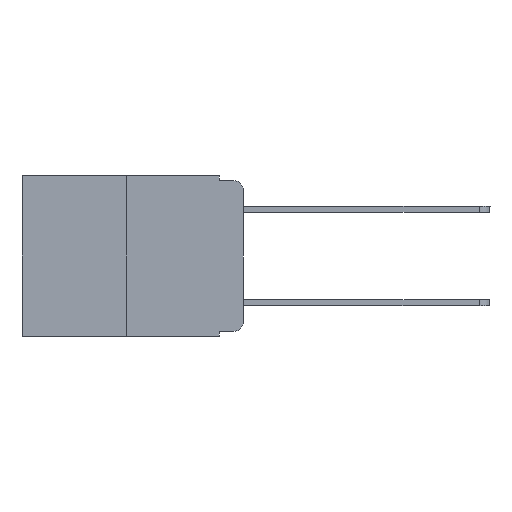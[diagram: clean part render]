
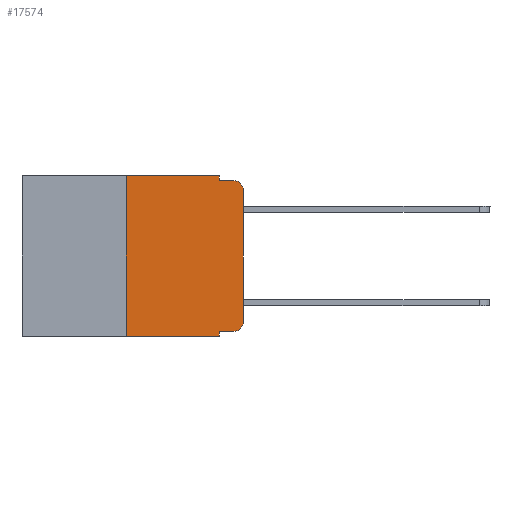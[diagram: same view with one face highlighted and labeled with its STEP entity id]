
A CAD part, left-side view. The second image highlights one B-rep face of the part: STEP entity #17574.
In plain terms, the highlighted planar face has unit normal (-1, 0, 0).
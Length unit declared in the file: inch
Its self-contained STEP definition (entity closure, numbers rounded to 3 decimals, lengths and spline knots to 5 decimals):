
#331 = EDGE_CURVE ( 'NONE', #4252, #5322, #2284, .T. ) ;
#807 = CARTESIAN_POINT ( 'NONE',  ( 0., 0.25, 0. ) ) ;
#851 = EDGE_CURVE ( 'NONE', #12747, #7354, #23218, .T. ) ;
#2124 = VERTEX_POINT ( 'NONE', #18488 ) ;
#2284 = LINE ( 'NONE', #20363, #13261 ) ;
#2447 = DIRECTION ( 'NONE',  ( 1., 0., 0. ) ) ;
#3952 = CARTESIAN_POINT ( 'NONE',  ( 0., 0.473, 0. ) ) ;
#4152 = EDGE_CURVE ( 'NONE', #25051, #7354, #22357, .T. ) ;
#4252 = VERTEX_POINT ( 'NONE', #8072 ) ;
#4361 = ORIENTED_EDGE ( 'NONE', *, *, #22997, .T. ) ;
#4567 = CIRCLE ( 'NONE', #19633, 0.02 ) ;
#4842 = ORIENTED_EDGE ( 'NONE', *, *, #851, .F. ) ;
#4973 = LINE ( 'NONE', #807, #24078 ) ;
#5035 = EDGE_CURVE ( 'NONE', #2124, #22050, #17595, .T. ) ;
#5322 = VERTEX_POINT ( 'NONE', #6813 ) ;
#5369 = DIRECTION ( 'NONE',  ( 0., -1., 0. ) ) ;
#6044 = CARTESIAN_POINT ( 'NONE',  ( 0., 0.051, -0.333 ) ) ;
#6506 = VERTEX_POINT ( 'NONE', #17336 ) ;
#6664 = VERTEX_POINT ( 'NONE', #6044 ) ;
#6665 = DIRECTION ( 'NONE',  ( 0., 0., 1. ) ) ;
#6740 = FACE_OUTER_BOUND ( 'NONE', #7889, .T. ) ;
#6813 = CARTESIAN_POINT ( 'NONE',  ( 0., 0.051, -0.343 ) ) ;
#6892 = ORIENTED_EDGE ( 'NONE', *, *, #12674, .F. ) ;
#7354 = VERTEX_POINT ( 'NONE', #19375 ) ;
#7362 = CARTESIAN_POINT ( 'NONE',  ( 0., 0.02, -0.333 ) ) ;
#7423 = DIRECTION ( 'NONE',  ( 0., 0., 1. ) ) ;
#7484 = ORIENTED_EDGE ( 'NONE', *, *, #12134, .F. ) ;
#7503 = VECTOR ( 'NONE', #5369, 39.37008 ) ;
#7889 = EDGE_LOOP ( 'NONE', ( #4361, #16773, #4842, #18980, #21516, #7484, #25048, #6892, #12847, #23120 ) ) ;
#8072 = CARTESIAN_POINT ( 'NONE',  ( 0., 0.25, -0.343 ) ) ;
#8151 = VECTOR ( 'NONE', #14756, 39.37008 ) ;
#8222 = LINE ( 'NONE', #10553, #11292 ) ;
#8453 = EDGE_CURVE ( 'NONE', #6664, #16986, #21256, .T. ) ;
#8575 = CARTESIAN_POINT ( 'NONE',  ( 0., 0.473, 0. ) ) ;
#8596 = CARTESIAN_POINT ( 'NONE',  ( 0., 0.051, 0. ) ) ;
#9507 = VECTOR ( 'NONE', #17309, 39.37008 ) ;
#10553 = CARTESIAN_POINT ( 'NONE',  ( 0., 0.051, 0. ) ) ;
#10653 = DIRECTION ( 'NONE',  ( -1., 0., 0. ) ) ;
#11100 = AXIS2_PLACEMENT_3D ( 'NONE', #8575, #2447, #12362 ) ;
#11216 = EDGE_CURVE ( 'NONE', #22050, #12747, #8222, .T. ) ;
#11217 = DIRECTION ( 'NONE',  ( -1., 0., 0. ) ) ;
#11292 = VECTOR ( 'NONE', #18573, 39.37008 ) ;
#12134 = EDGE_CURVE ( 'NONE', #4252, #2124, #4973, .T. ) ;
#12362 = DIRECTION ( 'NONE',  ( 0., 0., -1. ) ) ;
#12674 = EDGE_CURVE ( 'NONE', #6664, #5322, #14498, .T. ) ;
#12747 = VERTEX_POINT ( 'NONE', #16845 ) ;
#12847 = ORIENTED_EDGE ( 'NONE', *, *, #8453, .T. ) ;
#13216 = CARTESIAN_POINT ( 'NONE',  ( 0., 0.051, -0.01 ) ) ;
#13261 = VECTOR ( 'NONE', #14175, 39.37008 ) ;
#13437 = CARTESIAN_POINT ( 'NONE',  ( 0., 0., 0. ) ) ;
#13976 = VECTOR ( 'NONE', #25578, 39.37008 ) ;
#14175 = DIRECTION ( 'NONE',  ( 0., -1., 0. ) ) ;
#14498 = LINE ( 'NONE', #8596, #8151 ) ;
#14756 = DIRECTION ( 'NONE',  ( 0., 0., -1. ) ) ;
#14854 = DIRECTION ( 'NONE',  ( 0., 0., -1. ) ) ;
#15276 = CARTESIAN_POINT ( 'NONE',  ( 0., 0.051, 0. ) ) ;
#15465 = VECTOR ( 'NONE', #7423, 39.37008 ) ;
#16773 = ORIENTED_EDGE ( 'NONE', *, *, #4152, .T. ) ;
#16845 = CARTESIAN_POINT ( 'NONE',  ( 0., 0.051, -0.01 ) ) ;
#16986 = VERTEX_POINT ( 'NONE', #7362 ) ;
#17309 = DIRECTION ( 'NONE',  ( 0., -1., 0. ) ) ;
#17336 = CARTESIAN_POINT ( 'NONE',  ( 0., 0., -0.313 ) ) ;
#17574 = ADVANCED_FACE ( 'NONE', ( #6740 ), #20525, .F. ) ;
#17595 = LINE ( 'NONE', #3952, #13976 ) ;
#18488 = CARTESIAN_POINT ( 'NONE',  ( 0., 0.25, 0. ) ) ;
#18573 = DIRECTION ( 'NONE',  ( 0., 0., -1. ) ) ;
#18980 = ORIENTED_EDGE ( 'NONE', *, *, #11216, .F. ) ;
#19246 = DIRECTION ( 'NONE',  ( 0., 0., -1. ) ) ;
#19375 = CARTESIAN_POINT ( 'NONE',  ( 0., 0.02, -0.01 ) ) ;
#19633 = AXIS2_PLACEMENT_3D ( 'NONE', #22877, #10653, #14854 ) ;
#20257 = AXIS2_PLACEMENT_3D ( 'NONE', #23188, #11217, #19246 ) ;
#20363 = CARTESIAN_POINT ( 'NONE',  ( 0., 0.473, -0.343 ) ) ;
#20525 = PLANE ( 'NONE',  #11100 ) ;
#21256 = LINE ( 'NONE', #25554, #9507 ) ;
#21516 = ORIENTED_EDGE ( 'NONE', *, *, #5035, .F. ) ;
#22050 = VERTEX_POINT ( 'NONE', #15276 ) ;
#22288 = EDGE_CURVE ( 'NONE', #16986, #6506, #4567, .T. ) ;
#22357 = CIRCLE ( 'NONE', #20257, 0.02 ) ;
#22877 = CARTESIAN_POINT ( 'NONE',  ( 0., 0.02, -0.313 ) ) ;
#22997 = EDGE_CURVE ( 'NONE', #6506, #25051, #25377, .T. ) ;
#22998 = CARTESIAN_POINT ( 'NONE',  ( 0., 0., -0.03 ) ) ;
#23120 = ORIENTED_EDGE ( 'NONE', *, *, #22288, .T. ) ;
#23188 = CARTESIAN_POINT ( 'NONE',  ( 0., 0.02, -0.03 ) ) ;
#23218 = LINE ( 'NONE', #13216, #7503 ) ;
#24078 = VECTOR ( 'NONE', #6665, 39.37008 ) ;
#25048 = ORIENTED_EDGE ( 'NONE', *, *, #331, .T. ) ;
#25051 = VERTEX_POINT ( 'NONE', #22998 ) ;
#25377 = LINE ( 'NONE', #13437, #15465 ) ;
#25554 = CARTESIAN_POINT ( 'NONE',  ( 0., 0.051, -0.333 ) ) ;
#25578 = DIRECTION ( 'NONE',  ( 0., -1., 0. ) ) ;
